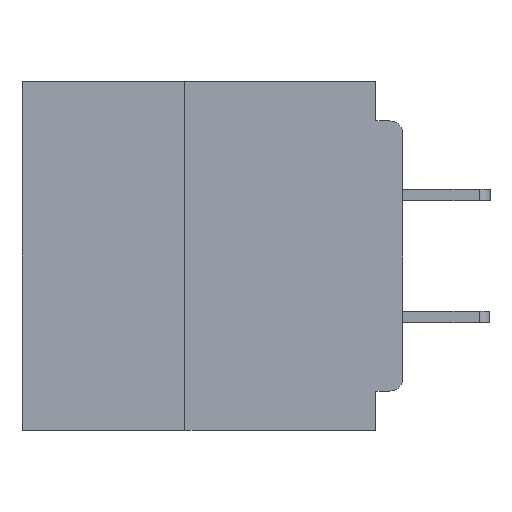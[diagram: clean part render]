
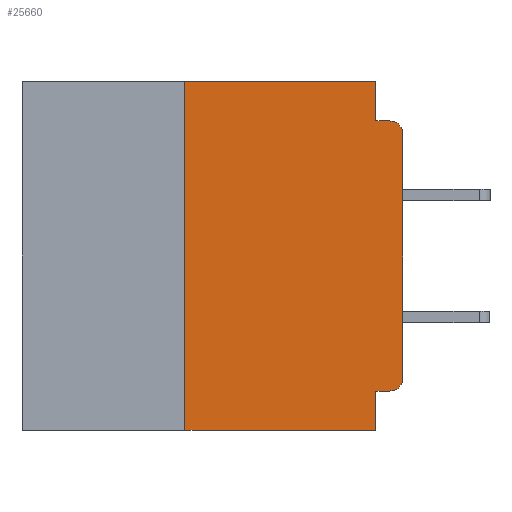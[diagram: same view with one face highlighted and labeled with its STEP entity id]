
A CAD part, left-side view. The second image highlights one B-rep face of the part: STEP entity #25660.
In plain terms, the highlighted planar face has unit normal (-1, 0, 0).
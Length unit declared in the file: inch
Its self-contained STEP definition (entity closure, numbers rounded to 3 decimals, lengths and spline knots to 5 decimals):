
#822 = VERTEX_POINT ( 'NONE', #3271 ) ;
#857 = ORIENTED_EDGE ( 'NONE', *, *, #38007, .T. ) ;
#903 = LINE ( 'NONE', #19743, #24064 ) ;
#1816 = ORIENTED_EDGE ( 'NONE', *, *, #3002, .T. ) ;
#2261 = LINE ( 'NONE', #28725, #18369 ) ;
#3002 = EDGE_CURVE ( 'NONE', #8928, #6950, #37468, .T. ) ;
#3225 = FACE_OUTER_BOUND ( 'NONE', #12001, .T. ) ;
#3271 = CARTESIAN_POINT ( 'NONE',  ( 0., 0.25, 0. ) ) ;
#3614 = VERTEX_POINT ( 'NONE', #25735 ) ;
#4134 = CARTESIAN_POINT ( 'NONE',  ( 0., 0.437, -0.4 ) ) ;
#4212 = VERTEX_POINT ( 'NONE', #18941 ) ;
#4264 = EDGE_CURVE ( 'NONE', #3614, #8928, #16244, .T. ) ;
#4484 = PLANE ( 'NONE',  #7027 ) ;
#6700 = VERTEX_POINT ( 'NONE', #20252 ) ;
#6838 = VECTOR ( 'NONE', #19213, 39.37008 ) ;
#6950 = VERTEX_POINT ( 'NONE', #38651 ) ;
#7027 = AXIS2_PLACEMENT_3D ( 'NONE', #25570, #28601, #10590 ) ;
#7623 = VERTEX_POINT ( 'NONE', #15751 ) ;
#7794 = LINE ( 'NONE', #4134, #6838 ) ;
#8928 = VERTEX_POINT ( 'NONE', #9359 ) ;
#9359 = CARTESIAN_POINT ( 'NONE',  ( 0., 0., -0.06 ) ) ;
#9573 = EDGE_CURVE ( 'NONE', #15866, #6700, #14009, .T. ) ;
#9671 = DIRECTION ( 'NONE',  ( 0., 0., 1. ) ) ;
#9771 = CARTESIAN_POINT ( 'NONE',  ( 0., 0.031, -0.4 ) ) ;
#9830 = LINE ( 'NONE', #36696, #16896 ) ;
#10590 = DIRECTION ( 'NONE',  ( 0., 0., -1. ) ) ;
#11126 = EDGE_CURVE ( 'NONE', #4212, #15866, #22412, .T. ) ;
#11396 = CARTESIAN_POINT ( 'NONE',  ( 0., 0., -0.355 ) ) ;
#11398 = ORIENTED_EDGE ( 'NONE', *, *, #9573, .F. ) ;
#11532 = LINE ( 'NONE', #14431, #34511 ) ;
#12001 = EDGE_LOOP ( 'NONE', ( #16982, #1816, #16697, #16384, #30726, #25080, #28890, #11398, #13955, #857 ) ) ;
#13955 = ORIENTED_EDGE ( 'NONE', *, *, #11126, .F. ) ;
#14009 = LINE ( 'NONE', #9771, #21119 ) ;
#14431 = CARTESIAN_POINT ( 'NONE',  ( 0., 0., -0.045 ) ) ;
#15320 = VECTOR ( 'NONE', #29389, 39.37008 ) ;
#15452 = CARTESIAN_POINT ( 'NONE',  ( 0., 0.031, 0. ) ) ;
#15616 = EDGE_CURVE ( 'NONE', #16786, #6700, #7794, .T. ) ;
#15751 = CARTESIAN_POINT ( 'NONE',  ( 0., 0.031, -0.045 ) ) ;
#15866 = VERTEX_POINT ( 'NONE', #20526 ) ;
#16244 = LINE ( 'NONE', #20260, #34093 ) ;
#16384 = ORIENTED_EDGE ( 'NONE', *, *, #25698, .F. ) ;
#16697 = ORIENTED_EDGE ( 'NONE', *, *, #29251, .F. ) ;
#16786 = VERTEX_POINT ( 'NONE', #34307 ) ;
#16896 = VECTOR ( 'NONE', #9671, 39.37008 ) ;
#16982 = ORIENTED_EDGE ( 'NONE', *, *, #4264, .T. ) ;
#17965 = CARTESIAN_POINT ( 'NONE',  ( 0., 0.015, -0.34 ) ) ;
#18369 = VECTOR ( 'NONE', #34590, 39.37008 ) ;
#18941 = CARTESIAN_POINT ( 'NONE',  ( 0., 0.015, -0.355 ) ) ;
#19213 = DIRECTION ( 'NONE',  ( 0., -1., 0. ) ) ;
#19290 = DIRECTION ( 'NONE',  ( 0., 0., 1. ) ) ;
#19743 = CARTESIAN_POINT ( 'NONE',  ( 0., 0.437, 0. ) ) ;
#20252 = CARTESIAN_POINT ( 'NONE',  ( 0., 0.031, -0.4 ) ) ;
#20260 = CARTESIAN_POINT ( 'NONE',  ( 0., 0., 0. ) ) ;
#20526 = CARTESIAN_POINT ( 'NONE',  ( 0., 0.031, -0.355 ) ) ;
#20536 = DIRECTION ( 'NONE',  ( 0., -1., 0. ) ) ;
#21009 = DIRECTION ( 'NONE',  ( 0., 0., -1. ) ) ;
#21119 = VECTOR ( 'NONE', #33791, 39.37008 ) ;
#21849 = AXIS2_PLACEMENT_3D ( 'NONE', #35158, #35127, #35118 ) ;
#22412 = LINE ( 'NONE', #11396, #15320 ) ;
#23610 = CIRCLE ( 'NONE', #29297, 0.015 ) ;
#23703 = EDGE_CURVE ( 'NONE', #16786, #822, #9830, .T. ) ;
#24064 = VECTOR ( 'NONE', #37664, 39.37008 ) ;
#25080 = ORIENTED_EDGE ( 'NONE', *, *, #23703, .F. ) ;
#25570 = CARTESIAN_POINT ( 'NONE',  ( 0., 0.437, 0. ) ) ;
#25660 = ADVANCED_FACE ( 'NONE', ( #3225 ), #4484, .F. ) ;
#25698 = EDGE_CURVE ( 'NONE', #29492, #7623, #2261, .T. ) ;
#25735 = CARTESIAN_POINT ( 'NONE',  ( 0., 0., -0.34 ) ) ;
#28601 = DIRECTION ( 'NONE',  ( 1., 0., 0. ) ) ;
#28725 = CARTESIAN_POINT ( 'NONE',  ( 0., 0.031, 0. ) ) ;
#28890 = ORIENTED_EDGE ( 'NONE', *, *, #15616, .T. ) ;
#29251 = EDGE_CURVE ( 'NONE', #7623, #6950, #11532, .T. ) ;
#29297 = AXIS2_PLACEMENT_3D ( 'NONE', #17965, #38889, #21009 ) ;
#29389 = DIRECTION ( 'NONE',  ( 0., 1., 0. ) ) ;
#29492 = VERTEX_POINT ( 'NONE', #15452 ) ;
#30726 = ORIENTED_EDGE ( 'NONE', *, *, #32847, .F. ) ;
#32847 = EDGE_CURVE ( 'NONE', #822, #29492, #903, .T. ) ;
#33791 = DIRECTION ( 'NONE',  ( 0., 0., -1. ) ) ;
#34093 = VECTOR ( 'NONE', #19290, 39.37008 ) ;
#34307 = CARTESIAN_POINT ( 'NONE',  ( 0., 0.25, -0.4 ) ) ;
#34511 = VECTOR ( 'NONE', #20536, 39.37008 ) ;
#34590 = DIRECTION ( 'NONE',  ( 0., 0., -1. ) ) ;
#35118 = DIRECTION ( 'NONE',  ( 0., 0., -1. ) ) ;
#35127 = DIRECTION ( 'NONE',  ( -1., 0., 0. ) ) ;
#35158 = CARTESIAN_POINT ( 'NONE',  ( 0., 0.015, -0.06 ) ) ;
#36696 = CARTESIAN_POINT ( 'NONE',  ( 0., 0.25, -0.4 ) ) ;
#37468 = CIRCLE ( 'NONE', #21849, 0.015 ) ;
#37664 = DIRECTION ( 'NONE',  ( 0., -1., 0. ) ) ;
#38007 = EDGE_CURVE ( 'NONE', #4212, #3614, #23610, .T. ) ;
#38651 = CARTESIAN_POINT ( 'NONE',  ( 0., 0.015, -0.045 ) ) ;
#38889 = DIRECTION ( 'NONE',  ( -1., 0., 0. ) ) ;
